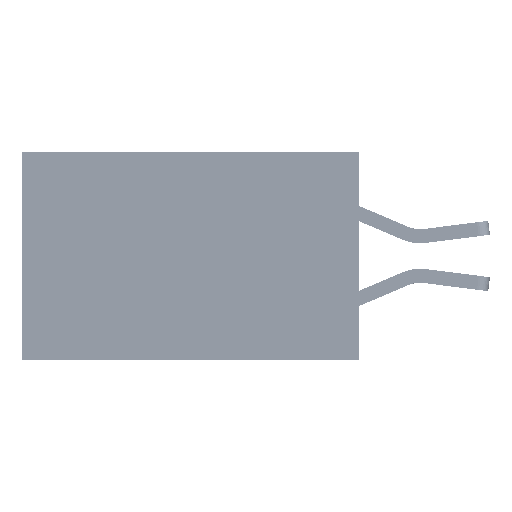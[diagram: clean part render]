
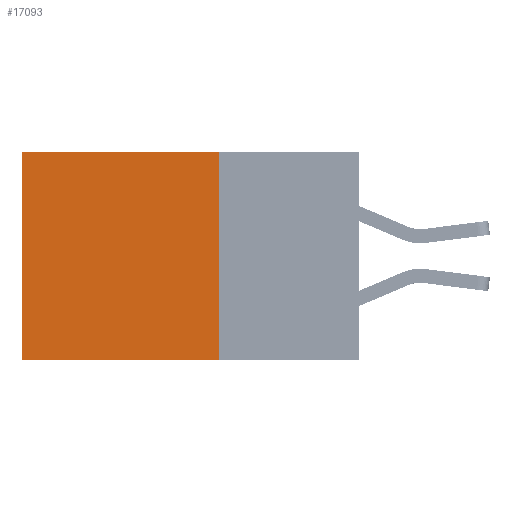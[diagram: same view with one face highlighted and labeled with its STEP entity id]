
A CAD part, left-side view. The second image highlights one B-rep face of the part: STEP entity #17093.
In plain terms, the highlighted planar face has unit normal (-1, 0, 0).
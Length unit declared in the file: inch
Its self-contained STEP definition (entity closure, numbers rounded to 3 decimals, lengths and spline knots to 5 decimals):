
#421 = DIRECTION ( 'NONE',  ( 0., 1., 0. ) ) ;
#1590 = DIRECTION ( 'NONE',  ( 0., 0., -1. ) ) ;
#4255 = VERTEX_POINT ( 'NONE', #17625 ) ;
#4996 = ORIENTED_EDGE ( 'NONE', *, *, #5875, .T. ) ;
#5875 = EDGE_CURVE ( 'NONE', #18702, #32429, #33022, .T. ) ;
#5979 = VECTOR ( 'NONE', #27359, 39.37008 ) ;
#6189 = EDGE_CURVE ( 'NONE', #20989, #18702, #32059, .T. ) ;
#7377 = VECTOR ( 'NONE', #8701, 39.37008 ) ;
#8093 = DIRECTION ( 'NONE',  ( 0., 0., -1. ) ) ;
#8701 = DIRECTION ( 'NONE',  ( 0., 1., 0. ) ) ;
#11085 = AXIS2_PLACEMENT_3D ( 'NONE', #19317, #32109, #1590 ) ;
#11755 = CARTESIAN_POINT ( 'NONE',  ( 0.2875, 0.25, 0. ) ) ;
#11888 = CARTESIAN_POINT ( 'NONE',  ( 0.2875, 0.25, -0.37 ) ) ;
#13968 = FACE_OUTER_BOUND ( 'NONE', #31563, .T. ) ;
#14094 = CARTESIAN_POINT ( 'NONE',  ( 0.2875, 0.6, -0.37 ) ) ;
#14262 = ORIENTED_EDGE ( 'NONE', *, *, #36714, .F. ) ;
#16268 = PLANE ( 'NONE',  #11085 ) ;
#17093 = ADVANCED_FACE ( 'NONE', ( #13968 ), #16268, .F. ) ;
#17162 = ORIENTED_EDGE ( 'NONE', *, *, #6189, .T. ) ;
#17625 = CARTESIAN_POINT ( 'NONE',  ( 0.2875, 0.25, -0.37 ) ) ;
#18702 = VERTEX_POINT ( 'NONE', #22344 ) ;
#19070 = CARTESIAN_POINT ( 'NONE',  ( 0.2875, 0.25, 0. ) ) ;
#19317 = CARTESIAN_POINT ( 'NONE',  ( 0.2875, 0.25, 0. ) ) ;
#20989 = VERTEX_POINT ( 'NONE', #26197 ) ;
#22344 = CARTESIAN_POINT ( 'NONE',  ( 0.2875, 0.6, 0. ) ) ;
#22649 = VECTOR ( 'NONE', #8093, 39.37008 ) ;
#22811 = CARTESIAN_POINT ( 'NONE',  ( 0.2875, 0.6, 0. ) ) ;
#23025 = LINE ( 'NONE', #11755, #5979 ) ;
#25472 = VECTOR ( 'NONE', #421, 39.37008 ) ;
#26197 = CARTESIAN_POINT ( 'NONE',  ( 0.2875, 0.25, 0. ) ) ;
#27359 = DIRECTION ( 'NONE',  ( 0., 0., -1. ) ) ;
#31563 = EDGE_LOOP ( 'NONE', ( #4996, #14262, #37650, #17162 ) ) ;
#32059 = LINE ( 'NONE', #19070, #25472 ) ;
#32109 = DIRECTION ( 'NONE',  ( 1., 0., 0. ) ) ;
#32429 = VERTEX_POINT ( 'NONE', #14094 ) ;
#33022 = LINE ( 'NONE', #22811, #22649 ) ;
#36714 = EDGE_CURVE ( 'NONE', #4255, #32429, #39081, .T. ) ;
#36774 = EDGE_CURVE ( 'NONE', #20989, #4255, #23025, .T. ) ;
#37650 = ORIENTED_EDGE ( 'NONE', *, *, #36774, .F. ) ;
#39081 = LINE ( 'NONE', #11888, #7377 ) ;
